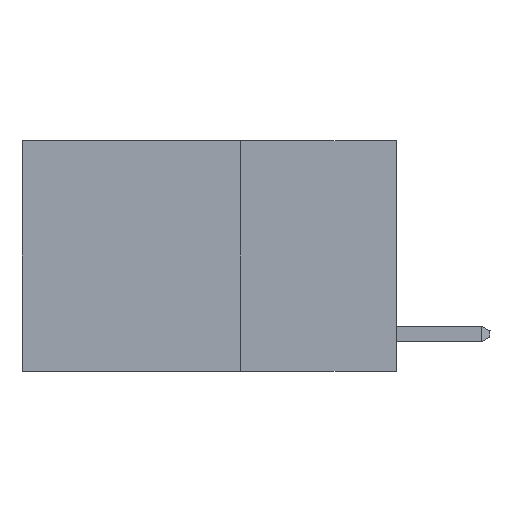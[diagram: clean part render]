
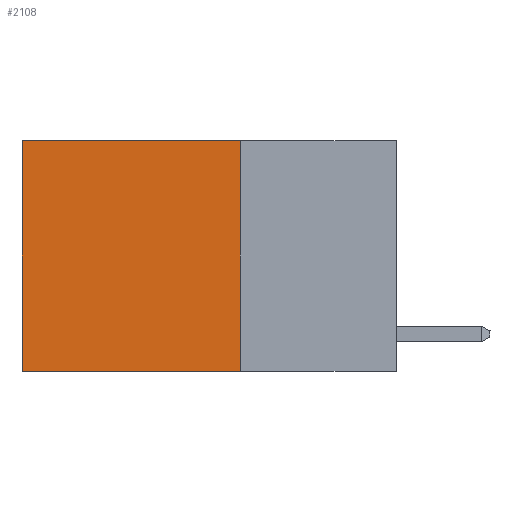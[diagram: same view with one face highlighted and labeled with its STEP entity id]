
A CAD part, left-side view. The second image highlights one B-rep face of the part: STEP entity #2108.
In plain terms, the highlighted planar face has unit normal (-1, 0, 0).
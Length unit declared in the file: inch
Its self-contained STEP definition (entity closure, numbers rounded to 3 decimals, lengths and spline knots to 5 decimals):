
#321 = VECTOR ( 'NONE', #14415, 39.37008 ) ;
#773 = VERTEX_POINT ( 'NONE', #22882 ) ;
#1588 = VECTOR ( 'NONE', #20164, 39.37008 ) ;
#2108 = ADVANCED_FACE ( 'NONE', ( #2840 ), #23989, .F. ) ;
#2661 = EDGE_CURVE ( 'NONE', #10274, #773, #3406, .T. ) ;
#2840 = FACE_OUTER_BOUND ( 'NONE', #24623, .T. ) ;
#2943 = CARTESIAN_POINT ( 'NONE',  ( 0.2625, 0.25, 0. ) ) ;
#3033 = CARTESIAN_POINT ( 'NONE',  ( 0.2625, 0.25, 0. ) ) ;
#3189 = ORIENTED_EDGE ( 'NONE', *, *, #2661, .T. ) ;
#3406 = LINE ( 'NONE', #14940, #23673 ) ;
#3985 = ORIENTED_EDGE ( 'NONE', *, *, #4736, .F. ) ;
#4238 = ORIENTED_EDGE ( 'NONE', *, *, #5449, .F. ) ;
#4736 = EDGE_CURVE ( 'NONE', #17981, #7647, #24137, .T. ) ;
#5449 = EDGE_CURVE ( 'NONE', #10274, #17981, #10760, .T. ) ;
#6580 = CARTESIAN_POINT ( 'NONE',  ( 0.2625, 0.25, 0. ) ) ;
#6778 = DIRECTION ( 'NONE',  ( 0., 0., -1. ) ) ;
#6823 = CARTESIAN_POINT ( 'NONE',  ( 0.2625, 0.25, -0.37 ) ) ;
#7426 = LINE ( 'NONE', #16261, #16094 ) ;
#7647 = VERTEX_POINT ( 'NONE', #16890 ) ;
#10274 = VERTEX_POINT ( 'NONE', #6580 ) ;
#10760 = LINE ( 'NONE', #3033, #1588 ) ;
#10805 = CARTESIAN_POINT ( 'NONE',  ( 0.2625, 0.25, -0.37 ) ) ;
#12739 = AXIS2_PLACEMENT_3D ( 'NONE', #2943, #14250, #6778 ) ;
#13085 = EDGE_CURVE ( 'NONE', #773, #7647, #7426, .T. ) ;
#14250 = DIRECTION ( 'NONE',  ( 1., 0., 0. ) ) ;
#14415 = DIRECTION ( 'NONE',  ( 0., 1., 0. ) ) ;
#14940 = CARTESIAN_POINT ( 'NONE',  ( 0.2625, 0.25, 0. ) ) ;
#16094 = VECTOR ( 'NONE', #23982, 39.37008 ) ;
#16261 = CARTESIAN_POINT ( 'NONE',  ( 0.2625, 0.6, 0. ) ) ;
#16890 = CARTESIAN_POINT ( 'NONE',  ( 0.2625, 0.6, -0.37 ) ) ;
#17981 = VERTEX_POINT ( 'NONE', #6823 ) ;
#20164 = DIRECTION ( 'NONE',  ( 0., 0., -1. ) ) ;
#22124 = ORIENTED_EDGE ( 'NONE', *, *, #13085, .T. ) ;
#22882 = CARTESIAN_POINT ( 'NONE',  ( 0.2625, 0.6, 0. ) ) ;
#23673 = VECTOR ( 'NONE', #24158, 39.37008 ) ;
#23982 = DIRECTION ( 'NONE',  ( 0., 0., -1. ) ) ;
#23989 = PLANE ( 'NONE',  #12739 ) ;
#24137 = LINE ( 'NONE', #10805, #321 ) ;
#24158 = DIRECTION ( 'NONE',  ( 0., 1., 0. ) ) ;
#24623 = EDGE_LOOP ( 'NONE', ( #22124, #3985, #4238, #3189 ) ) ;
